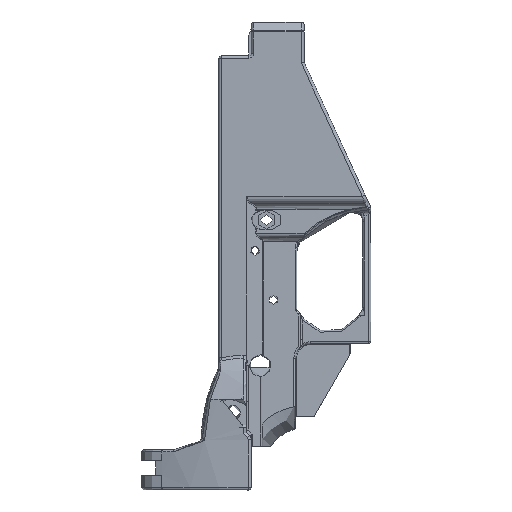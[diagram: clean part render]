
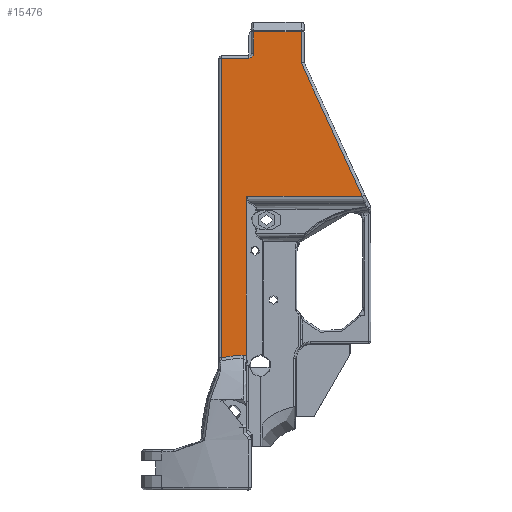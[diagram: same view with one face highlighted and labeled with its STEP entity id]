
A CAD part, left-side view. The second image highlights one B-rep face of the part: STEP entity #15476.
In plain terms, the highlighted planar face has unit normal (-1, 0, 0).
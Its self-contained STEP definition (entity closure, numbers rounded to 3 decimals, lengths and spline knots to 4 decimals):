
#219=ELLIPSE('',#16877,1.9201,1.636);
#397=PLANE('',#16875);
#1354=FACE_OUTER_BOUND('',#2304,.T.);
#2304=EDGE_LOOP('',(#12503,#12504,#12505,#12506,#12507,#12508,#12509,#12510,
#12511,#12512,#12513,#12514));
#3249=B_SPLINE_CURVE_WITH_KNOTS('',3,(#43629,#43630,#43631,#43632),
 .UNSPECIFIED.,.F.,.F.,(4,4),(-0.1434,0.),
 .UNSPECIFIED.);
#3250=B_SPLINE_CURVE_WITH_KNOTS('',3,(#43636,#43637,#43638,#43639,#43640,
#43641,#43642,#43643,#43644,#43645,#43646,#43647),.UNSPECIFIED.,.F.,.F.,
(4,2,2,2,2,4),(-0.117,-0.1147,-0.0798,
-0.057,-0.0072,0.),.UNSPECIFIED.);
#3883=CIRCLE('',#16876,0.08);
#4504=LINE('',#26158,#5273);
#4506=LINE('',#26189,#5275);
#4686=LINE('',#43581,#5455);
#4690=LINE('',#43619,#5459);
#4691=LINE('',#43623,#5460);
#4692=LINE('',#43625,#5461);
#4693=LINE('',#43634,#5462);
#4694=LINE('',#43648,#5463);
#5273=VECTOR('',#19110,0.3937);
#5275=VECTOR('',#19122,0.3937);
#5455=VECTOR('',#19952,0.3937);
#5459=VECTOR('',#19974,0.3937);
#5460=VECTOR('',#19977,0.3937);
#5461=VECTOR('',#19978,0.3937);
#5462=VECTOR('',#19981,1.6985);
#5463=VECTOR('',#19982,0.1181);
#6288=VERTEX_POINT('',#26155);
#6289=VERTEX_POINT('',#26157);
#6293=VERTEX_POINT('',#26187);
#6797=VERTEX_POINT('',#43579);
#6802=VERTEX_POINT('',#43618);
#6803=VERTEX_POINT('',#43620);
#6804=VERTEX_POINT('',#43622);
#6805=VERTEX_POINT('',#43624);
#6806=VERTEX_POINT('',#43626);
#6807=VERTEX_POINT('',#43628);
#6808=VERTEX_POINT('',#43633);
#6809=VERTEX_POINT('',#43635);
#8083=EDGE_CURVE('',#6288,#6289,#4504,.T.);
#8090=EDGE_CURVE('',#6293,#6288,#4506,.T.);
#8826=EDGE_CURVE('',#6797,#6293,#4686,.T.);
#8835=EDGE_CURVE('',#6802,#6797,#4690,.T.);
#8836=EDGE_CURVE('',#6803,#6802,#3883,.T.);
#8837=EDGE_CURVE('',#6804,#6803,#4691,.T.);
#8838=EDGE_CURVE('',#6805,#6804,#4692,.T.);
#8839=EDGE_CURVE('',#6806,#6805,#219,.T.);
#8840=EDGE_CURVE('',#6807,#6806,#3249,.T.);
#8841=EDGE_CURVE('',#6808,#6807,#4693,.T.);
#8842=EDGE_CURVE('',#6809,#6808,#3250,.T.);
#8843=EDGE_CURVE('',#6289,#6809,#4694,.T.);
#12503=ORIENTED_EDGE('',*,*,#8083,.F.);
#12504=ORIENTED_EDGE('',*,*,#8090,.F.);
#12505=ORIENTED_EDGE('',*,*,#8826,.F.);
#12506=ORIENTED_EDGE('',*,*,#8835,.F.);
#12507=ORIENTED_EDGE('',*,*,#8836,.F.);
#12508=ORIENTED_EDGE('',*,*,#8837,.F.);
#12509=ORIENTED_EDGE('',*,*,#8838,.F.);
#12510=ORIENTED_EDGE('',*,*,#8839,.F.);
#12511=ORIENTED_EDGE('',*,*,#8840,.F.);
#12512=ORIENTED_EDGE('',*,*,#8841,.F.);
#12513=ORIENTED_EDGE('',*,*,#8842,.F.);
#12514=ORIENTED_EDGE('',*,*,#8843,.F.);
#15476=ADVANCED_FACE('',(#1354),#397,.F.);
#16875=AXIS2_PLACEMENT_3D('',#43617,#19972,#19973);
#16876=AXIS2_PLACEMENT_3D('',#43621,#19975,#19976);
#16877=AXIS2_PLACEMENT_3D('',#43627,#19979,#19980);
#19110=DIRECTION('',(0.,-0.417,-0.909));
#19122=DIRECTION('',(0.,0.,-1.));
#19952=DIRECTION('',(0.,-1.,0.));
#19972=DIRECTION('center_axis',(1.,0.,0.));
#19973=DIRECTION('ref_axis',(0.,0.,
-1.));
#19974=DIRECTION('',(0.,0.,1.));
#19975=DIRECTION('center_axis',(-1.,0.,0.));
#19976=DIRECTION('ref_axis',(0.,-0.707,-0.707));
#19977=DIRECTION('',(0.,-1.,0.));
#19978=DIRECTION('',(0.,0.,1.));
#19979=DIRECTION('center_axis',(-1.,0.,0.));
#19980=DIRECTION('ref_axis',(0.,-0.984,-0.179));
#19981=DIRECTION('',(0.,0.,-1.));
#19982=DIRECTION('',(0.,1.,0.));
#26155=CARTESIAN_POINT('',(-0.731,-0.0727,2.8507));
#26157=CARTESIAN_POINT('',(-0.731,-1.118,0.5717));
#26158=CARTESIAN_POINT('',(-0.731,-1.4648,-0.1846));
#26187=CARTESIAN_POINT('',(-0.731,-0.0728,3.3816));
#26189=CARTESIAN_POINT('',(-0.731,-0.0727,-0.2092));
#43579=CARTESIAN_POINT('',(-0.731,0.7372,3.3816));
#43581=CARTESIAN_POINT('',(-0.731,0.7121,3.3816));
#43617=CARTESIAN_POINT('Origin',(-0.731,0.68,-3.6849));
#43618=CARTESIAN_POINT('',(-0.731,0.7373,3.0095));
#43619=CARTESIAN_POINT('',(-0.731,0.7373,-0.0118));
#43620=CARTESIAN_POINT('',(-0.731,0.8173,2.9295));
#43621=CARTESIAN_POINT('Origin',(-0.731,0.8173,3.0095));
#43622=CARTESIAN_POINT('',(-0.731,1.2902,2.9295));
#43623=CARTESIAN_POINT('',(-0.731,0.7441,2.9295));
#43624=CARTESIAN_POINT('',(-0.731,1.2902,-2.1813));
#43625=CARTESIAN_POINT('',(-0.731,1.2902,-3.1756));
#43626=CARTESIAN_POINT('',(-0.731,0.9158,-2.1342));
#43627=CARTESIAN_POINT('Origin',(-0.731,0.7244,-3.7785));
#43628=CARTESIAN_POINT('',(-0.731,0.8628,-2.151));
#43629=CARTESIAN_POINT('Ctrl Pts',(-0.731,0.8629,
-2.151));
#43630=CARTESIAN_POINT('Ctrl Pts',(-0.731,0.8784,
-2.1404));
#43631=CARTESIAN_POINT('Ctrl Pts',(-0.731,0.8969,
-2.1335));
#43632=CARTESIAN_POINT('Ctrl Pts',(-0.731,0.9158,
-2.1342));
#43633=CARTESIAN_POINT('',(-0.731,0.8628,0.5319));
#43634=CARTESIAN_POINT('',(-0.731,0.8628,-2.5001));
#43635=CARTESIAN_POINT('',(-0.731,0.8546,0.5717));
#43636=CARTESIAN_POINT('Ctrl Pts',(-0.731,0.8546,
0.5717));
#43637=CARTESIAN_POINT('Ctrl Pts',(-0.731,0.8546,
0.5716));
#43638=CARTESIAN_POINT('Ctrl Pts',(-0.731,0.8546,
0.5716));
#43639=CARTESIAN_POINT('Ctrl Pts',(-0.731,0.855,
0.5706));
#43640=CARTESIAN_POINT('Ctrl Pts',(-0.731,0.8564,
0.5674));
#43641=CARTESIAN_POINT('Ctrl Pts',(-0.731,0.8587,
0.5601));
#43642=CARTESIAN_POINT('Ctrl Pts',(-0.731,0.8595,
0.5572));
#43643=CARTESIAN_POINT('Ctrl Pts',(-0.731,0.8617,
0.5478));
#43644=CARTESIAN_POINT('Ctrl Pts',(-0.731,0.8626,
0.5413));
#43645=CARTESIAN_POINT('Ctrl Pts',(-0.731,0.8628,
0.5338));
#43646=CARTESIAN_POINT('Ctrl Pts',(-0.731,0.8628,
0.5329));
#43647=CARTESIAN_POINT('Ctrl Pts',(-0.731,0.8628,
0.5319));
#43648=CARTESIAN_POINT('',(-0.731,1.0895,0.5717));
